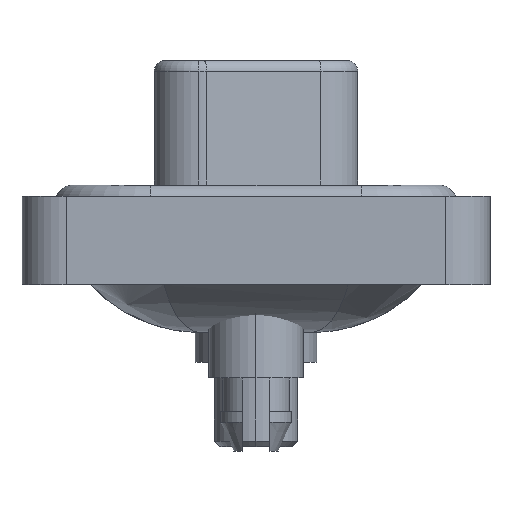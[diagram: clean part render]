
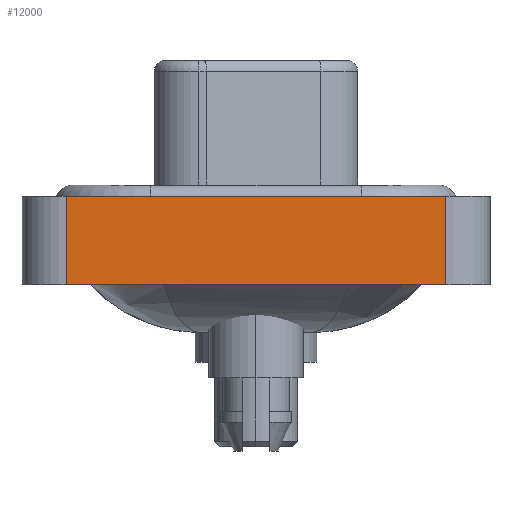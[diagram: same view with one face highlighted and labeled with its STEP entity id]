
A CAD part, left-side view. The second image highlights one B-rep face of the part: STEP entity #12000.
In plain terms, the highlighted planar face has unit normal (-1, 0, 0).
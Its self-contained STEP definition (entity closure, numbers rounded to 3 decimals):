
#133 = LINE ( 'NONE', #6796, #652 ) ;
#652 = VECTOR ( 'NONE', #14857, 1000. ) ;
#1109 = VERTEX_POINT ( 'NONE', #6037 ) ;
#1537 = ORIENTED_EDGE ( 'NONE', *, *, #10256, .F. ) ;
#2946 = EDGE_CURVE ( 'NONE', #1109, #10041, #133, .T. ) ;
#3344 = AXIS2_PLACEMENT_3D ( 'NONE', #11641, #17000, #14280 ) ;
#3924 = ORIENTED_EDGE ( 'NONE', *, *, #11411, .F. ) ;
#4348 = CARTESIAN_POINT ( 'NONE',  ( -7.3, -8.55, 0.4 ) ) ;
#4794 = DIRECTION ( 'NONE',  ( 0., 0., 1. ) ) ;
#5258 = EDGE_LOOP ( 'NONE', ( #11488, #3924, #1537, #8550 ) ) ;
#5609 = DIRECTION ( 'NONE',  ( 0., 0., 1. ) ) ;
#6037 = CARTESIAN_POINT ( 'NONE',  ( -7.3, 8.55, -3.6 ) ) ;
#6591 = VERTEX_POINT ( 'NONE', #14060 ) ;
#6796 = CARTESIAN_POINT ( 'NONE',  ( -7.3, -8.55, -3.6 ) ) ;
#7710 = PLANE ( 'NONE',  #3344 ) ;
#8550 = ORIENTED_EDGE ( 'NONE', *, *, #2946, .T. ) ;
#9704 = DIRECTION ( 'NONE',  ( 0., -1., 0. ) ) ;
#9979 = EDGE_CURVE ( 'NONE', #10041, #6591, #10603, .T. ) ;
#10041 = VERTEX_POINT ( 'NONE', #10965 ) ;
#10256 = EDGE_CURVE ( 'NONE', #1109, #16437, #11462, .T. ) ;
#10603 = LINE ( 'NONE', #17187, #11127 ) ;
#10965 = CARTESIAN_POINT ( 'NONE',  ( -7.3, -8.55, -3.6 ) ) ;
#11127 = VECTOR ( 'NONE', #5609, 1000. ) ;
#11411 = EDGE_CURVE ( 'NONE', #16437, #6591, #12423, .T. ) ;
#11462 = LINE ( 'NONE', #16816, #16727 ) ;
#11488 = ORIENTED_EDGE ( 'NONE', *, *, #9979, .T. ) ;
#11641 = CARTESIAN_POINT ( 'NONE',  ( -7.3, -8.55, -3.6 ) ) ;
#12000 = ADVANCED_FACE ( 'NONE', ( #15516 ), #7710, .T. ) ;
#12423 = LINE ( 'NONE', #4348, #13400 ) ;
#12475 = CARTESIAN_POINT ( 'NONE',  ( -7.3, 8.55, 0.4 ) ) ;
#13400 = VECTOR ( 'NONE', #9704, 1000. ) ;
#14060 = CARTESIAN_POINT ( 'NONE',  ( -7.3, -8.55, 0.4 ) ) ;
#14280 = DIRECTION ( 'NONE',  ( 0., 0., 1. ) ) ;
#14857 = DIRECTION ( 'NONE',  ( 0., -1., 0. ) ) ;
#15516 = FACE_OUTER_BOUND ( 'NONE', #5258, .T. ) ;
#16437 = VERTEX_POINT ( 'NONE', #12475 ) ;
#16727 = VECTOR ( 'NONE', #4794, 1000. ) ;
#16816 = CARTESIAN_POINT ( 'NONE',  ( -7.3, 8.55, -3.6 ) ) ;
#17000 = DIRECTION ( 'NONE',  ( -1., 0., 0. ) ) ;
#17187 = CARTESIAN_POINT ( 'NONE',  ( -7.3, -8.55, -3.6 ) ) ;
